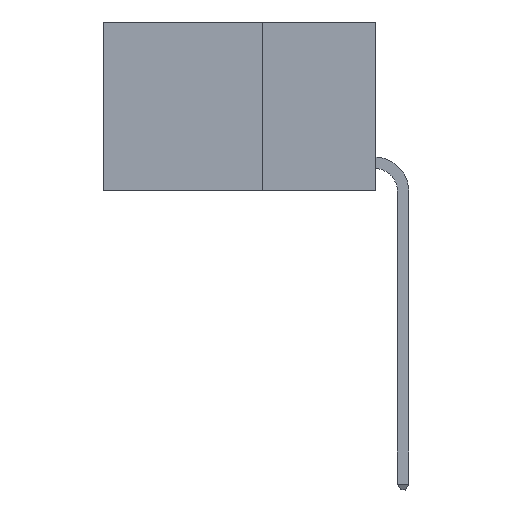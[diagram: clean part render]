
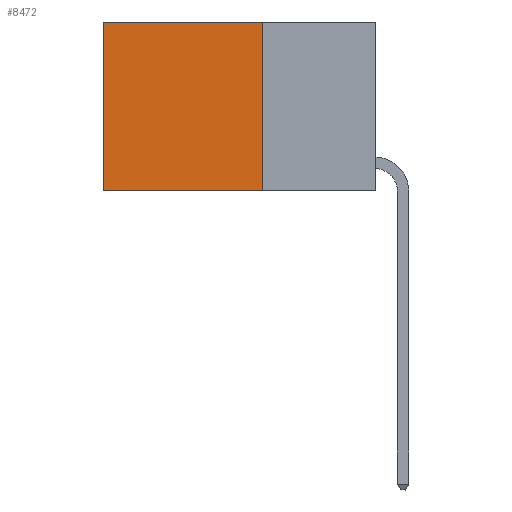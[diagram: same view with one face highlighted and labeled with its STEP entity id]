
A CAD part, left-side view. The second image highlights one B-rep face of the part: STEP entity #8472.
In plain terms, the highlighted planar face has unit normal (-1, 0, 0).
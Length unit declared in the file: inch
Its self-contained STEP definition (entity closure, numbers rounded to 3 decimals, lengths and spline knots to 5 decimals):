
#1548 = DIRECTION ( 'NONE',  ( 0., 0., -1. ) ) ;
#1617 = CARTESIAN_POINT ( 'NONE',  ( 0.2625, 0.6, -0.37 ) ) ;
#1732 = ORIENTED_EDGE ( 'NONE', *, *, #7987, .T. ) ;
#2350 = ORIENTED_EDGE ( 'NONE', *, *, #20305, .F. ) ;
#2828 = DIRECTION ( 'NONE',  ( 0., 0., -1. ) ) ;
#3723 = VECTOR ( 'NONE', #1548, 39.37008 ) ;
#4461 = VERTEX_POINT ( 'NONE', #1617 ) ;
#4479 = LINE ( 'NONE', #8755, #3723 ) ;
#4637 = VERTEX_POINT ( 'NONE', #31076 ) ;
#4913 = ORIENTED_EDGE ( 'NONE', *, *, #5336, .T. ) ;
#5336 = EDGE_CURVE ( 'NONE', #4637, #4461, #20413, .T. ) ;
#5464 = PLANE ( 'NONE',  #12447 ) ;
#7987 = EDGE_CURVE ( 'NONE', #8275, #4637, #20810, .T. ) ;
#8148 = DIRECTION ( 'NONE',  ( 0., 1., 0. ) ) ;
#8275 = VERTEX_POINT ( 'NONE', #16716 ) ;
#8413 = VECTOR ( 'NONE', #2828, 39.37008 ) ;
#8472 = ADVANCED_FACE ( 'NONE', ( #19246 ), #5464, .F. ) ;
#8755 = CARTESIAN_POINT ( 'NONE',  ( 0.2625, 0.25, 0. ) ) ;
#9078 = VERTEX_POINT ( 'NONE', #18253 ) ;
#9337 = CARTESIAN_POINT ( 'NONE',  ( 0.2625, 0.25, -0.37 ) ) ;
#10103 = CARTESIAN_POINT ( 'NONE',  ( 0.2625, 0.6, 0. ) ) ;
#12447 = AXIS2_PLACEMENT_3D ( 'NONE', #17449, #27166, #12709 ) ;
#12709 = DIRECTION ( 'NONE',  ( 0., 0., -1. ) ) ;
#14144 = ORIENTED_EDGE ( 'NONE', *, *, #21749, .F. ) ;
#14374 = VECTOR ( 'NONE', #8148, 39.37008 ) ;
#16716 = CARTESIAN_POINT ( 'NONE',  ( 0.2625, 0.25, 0. ) ) ;
#17449 = CARTESIAN_POINT ( 'NONE',  ( 0.2625, 0.25, 0. ) ) ;
#18253 = CARTESIAN_POINT ( 'NONE',  ( 0.2625, 0.25, -0.37 ) ) ;
#18305 = LINE ( 'NONE', #9337, #24716 ) ;
#19246 = FACE_OUTER_BOUND ( 'NONE', #22960, .T. ) ;
#20305 = EDGE_CURVE ( 'NONE', #8275, #9078, #4479, .T. ) ;
#20413 = LINE ( 'NONE', #10103, #8413 ) ;
#20810 = LINE ( 'NONE', #27388, #14374 ) ;
#21749 = EDGE_CURVE ( 'NONE', #9078, #4461, #18305, .T. ) ;
#22960 = EDGE_LOOP ( 'NONE', ( #4913, #14144, #2350, #1732 ) ) ;
#24716 = VECTOR ( 'NONE', #26167, 39.37008 ) ;
#26167 = DIRECTION ( 'NONE',  ( 0., 1., 0. ) ) ;
#27166 = DIRECTION ( 'NONE',  ( 1., 0., 0. ) ) ;
#27388 = CARTESIAN_POINT ( 'NONE',  ( 0.2625, 0.25, 0. ) ) ;
#31076 = CARTESIAN_POINT ( 'NONE',  ( 0.2625, 0.6, 0. ) ) ;
